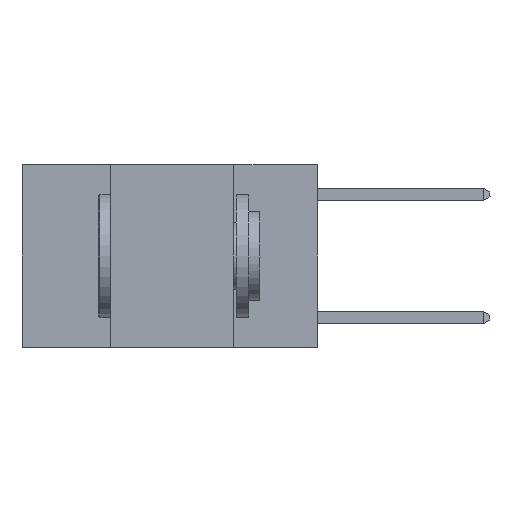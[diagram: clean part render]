
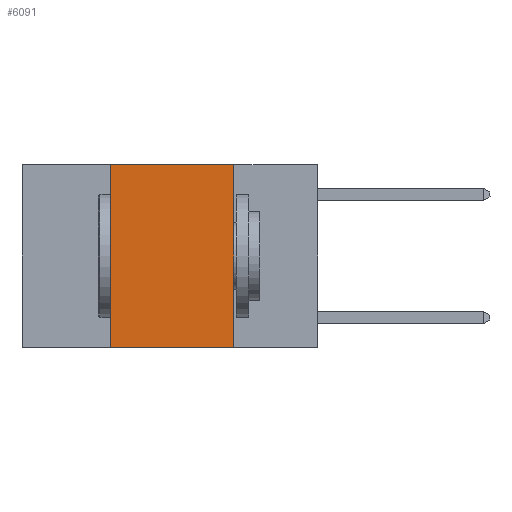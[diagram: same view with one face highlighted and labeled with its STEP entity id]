
A CAD part, left-side view. The second image highlights one B-rep face of the part: STEP entity #6091.
In plain terms, the highlighted planar face has unit normal (-1, 0, 0).
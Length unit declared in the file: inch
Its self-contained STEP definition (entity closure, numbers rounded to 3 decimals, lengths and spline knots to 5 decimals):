
#12 = FACE_OUTER_BOUND ( 'NONE', #3218, .T. ) ;
#473 = VECTOR ( 'NONE', #8625, 39.37008 ) ;
#908 = LINE ( 'NONE', #4660, #8585 ) ;
#1005 = VERTEX_POINT ( 'NONE', #6728 ) ;
#1729 = DIRECTION ( 'NONE',  ( 0., 0., -1. ) ) ;
#1819 = EDGE_CURVE ( 'NONE', #6573, #3865, #3602, .T. ) ;
#2137 = DIRECTION ( 'NONE',  ( 0., -1., 0. ) ) ;
#2249 = CARTESIAN_POINT ( 'NONE',  ( 0., 0.17, -0.37 ) ) ;
#2362 = CARTESIAN_POINT ( 'NONE',  ( 0., 0.42, 0. ) ) ;
#2506 = EDGE_CURVE ( 'NONE', #6573, #4765, #3193, .T. ) ;
#3193 = LINE ( 'NONE', #6915, #4450 ) ;
#3218 = EDGE_LOOP ( 'NONE', ( #6447, #7789, #8193, #5016 ) ) ;
#3418 = EDGE_CURVE ( 'NONE', #4765, #1005, #908, .T. ) ;
#3602 = LINE ( 'NONE', #5729, #3776 ) ;
#3776 = VECTOR ( 'NONE', #2137, 39.37008 ) ;
#3865 = VERTEX_POINT ( 'NONE', #2249 ) ;
#4100 = CARTESIAN_POINT ( 'NONE',  ( 0., 0.42, -0.37 ) ) ;
#4450 = VECTOR ( 'NONE', #7632, 39.37008 ) ;
#4660 = CARTESIAN_POINT ( 'NONE',  ( 0., 0.6, 0. ) ) ;
#4765 = VERTEX_POINT ( 'NONE', #2362 ) ;
#4984 = LINE ( 'NONE', #9123, #473 ) ;
#5016 = ORIENTED_EDGE ( 'NONE', *, *, #1819, .T. ) ;
#5158 = CARTESIAN_POINT ( 'NONE',  ( 0., 0.6, 0. ) ) ;
#5729 = CARTESIAN_POINT ( 'NONE',  ( 0., 0.6, -0.37 ) ) ;
#6091 = ADVANCED_FACE ( 'NONE', ( #12 ), #8327, .F. ) ;
#6447 = ORIENTED_EDGE ( 'NONE', *, *, #8764, .F. ) ;
#6573 = VERTEX_POINT ( 'NONE', #4100 ) ;
#6728 = CARTESIAN_POINT ( 'NONE',  ( 0., 0.17, 0. ) ) ;
#6915 = CARTESIAN_POINT ( 'NONE',  ( 0., 0.42, 0. ) ) ;
#7632 = DIRECTION ( 'NONE',  ( 0., 0., 1. ) ) ;
#7789 = ORIENTED_EDGE ( 'NONE', *, *, #3418, .F. ) ;
#8193 = ORIENTED_EDGE ( 'NONE', *, *, #2506, .F. ) ;
#8277 = AXIS2_PLACEMENT_3D ( 'NONE', #5158, #8801, #1729 ) ;
#8327 = PLANE ( 'NONE',  #8277 ) ;
#8585 = VECTOR ( 'NONE', #9062, 39.37008 ) ;
#8625 = DIRECTION ( 'NONE',  ( 0., 0., -1. ) ) ;
#8764 = EDGE_CURVE ( 'NONE', #1005, #3865, #4984, .T. ) ;
#8801 = DIRECTION ( 'NONE',  ( 1., 0., 0. ) ) ;
#9062 = DIRECTION ( 'NONE',  ( 0., -1., 0. ) ) ;
#9123 = CARTESIAN_POINT ( 'NONE',  ( 0., 0.17, 0. ) ) ;
